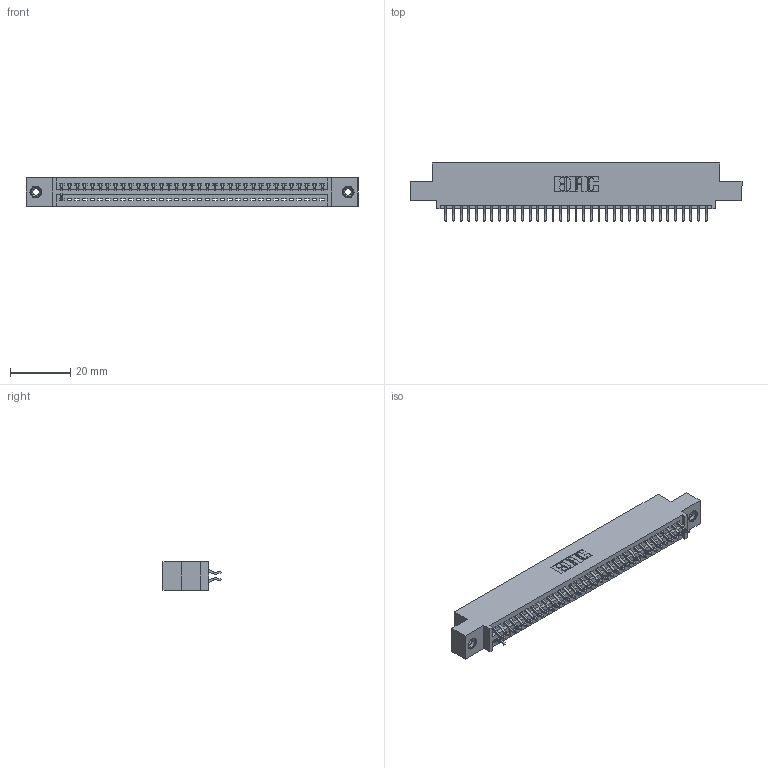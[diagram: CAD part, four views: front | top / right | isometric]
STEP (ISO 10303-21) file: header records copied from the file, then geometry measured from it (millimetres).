
FILE_DESCRIPTION (( 'STEP AP203' ), '1' );
FILE_NAME ('395-070-556-508.STEP', '2018-11-27T01:05:45', ( '' ), ( '' ), 'SwSTEP 2.0', 'SolidWorks 2016', '' );
FILE_SCHEMA (( 'CONFIG_CONTROL_DESIGN' ));
Length unit declared in the file: inch
Products named in the file (4): 345-250-001_345-250-003-102; 345-292-001_556 Tail; 395-070-556-508; 345 Part_0.110 Offset - 0.156 Dia-TI
Assembly tree (39 placements, depth 2):
  395-070-556-508
    345 Part_0.110 Offset - 0.156 Dia-TI
    345-292-001_556 Tail  x36
    345-250-001_345-250-003-102  x2
Bounding box: 110.11 x 19.24 x 9.4 mm (x, y, z)
Volume: 10243.3 mm3; surface area: 13344.7 mm2
Topology: 39 solids, 39 shells, 2478 faces, 7419 edges, 4890 vertices
Faces by surface type: plane 1686, cylinder 776, cone 12, torus 4
Entity records: 28854 total; most frequent: CARTESIAN_POINT 4989, ORIENTED_EDGE 4938, DIRECTION 4383, EDGE_CURVE 2469, VECTOR 2169, LINE 2169, VERTEX_POINT 1640, AXIS2_PLACEMENT_3D 1107
